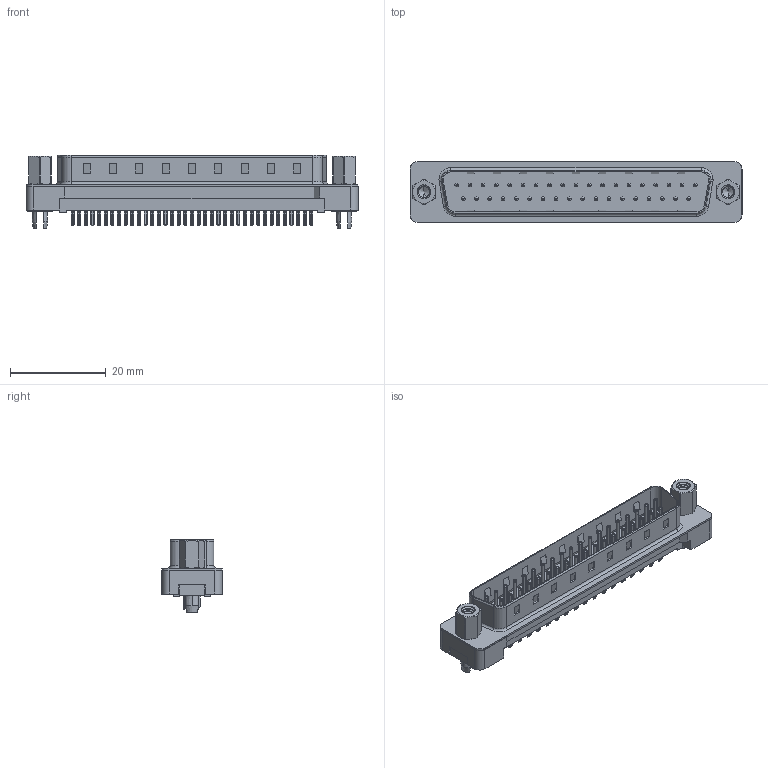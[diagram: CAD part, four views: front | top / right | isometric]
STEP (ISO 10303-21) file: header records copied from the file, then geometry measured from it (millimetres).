
FILE_DESCRIPTION (( 'STEP AP203' ), '1' );
FILE_NAME ('627-037-220-217.STEP', '2020-07-16T01:35:21', ( '' ), ( '' ), 'SwSTEP 2.0', 'SolidWorks 2020', '' );
FILE_SCHEMA (( 'CONFIG_CONTROL_DESIGN' ));
Length unit declared in the file: millimetre
Products named in the file (7): 627 PB Shell_37 Contacts; 627 Plastic Body Housing_37 Contacts; 627 4-40 Hex Standoff; 627 PB 4-40 Threaded Rivet with Boardlock; 627 PB Contact Row 1_20; 627-037-220-217; 627 PB Contact Row 2_20
Assembly tree (43 placements, depth 2):
  627-037-220-217
    627 Plastic Body Housing_37 Contacts
    627 PB Shell_37 Contacts
    627 PB Contact Row 1_20  x19
    627 PB Contact Row 2_20  x18
    627 4-40 Hex Standoff  x2
    627 PB 4-40 Threaded Rivet with Boardlock  x2
Bounding box: 69.32 x 12.6 x 15.25 mm (x, y, z)
Volume: 3445.5 mm3; surface area: 8131.9 mm2
Topology: 43 solids, 43 shells, 2629 faces, 6996 edges, 4503 vertices
Faces by surface type: plane 1673, cylinder 766, torus 130, cone 42, bspline 18
Entity records: 33530 total; most frequent: CARTESIAN_POINT 8548, ORIENTED_EDGE 4868, DIRECTION 4772, EDGE_CURVE 2434, LINE 1706, VECTOR 1706, VERTEX_POINT 1587, AXIS2_PLACEMENT_3D 1533
